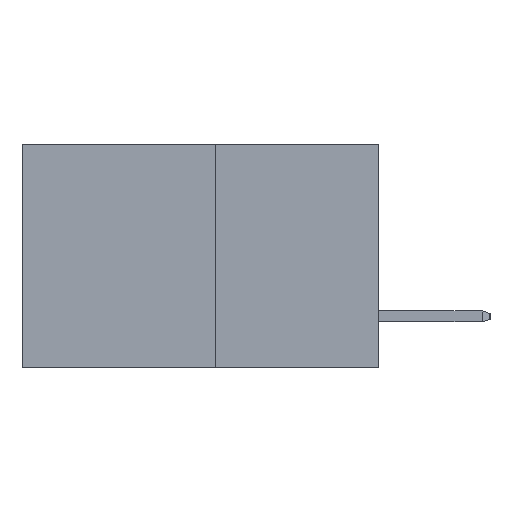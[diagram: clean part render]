
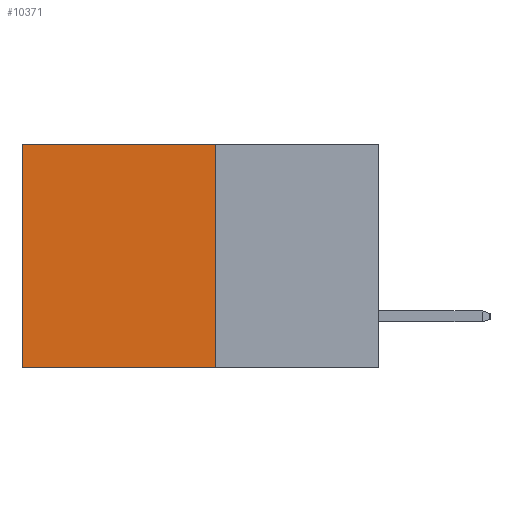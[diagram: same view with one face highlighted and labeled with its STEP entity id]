
A CAD part, left-side view. The second image highlights one B-rep face of the part: STEP entity #10371.
In plain terms, the highlighted planar face has unit normal (-1, 0, 0).
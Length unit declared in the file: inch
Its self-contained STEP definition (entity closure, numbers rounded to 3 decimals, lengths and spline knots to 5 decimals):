
#723 = EDGE_CURVE ( 'NONE', #2415, #3083, #956, .T. ) ;
#948 = VECTOR ( 'NONE', #29250, 39.37008 ) ;
#956 = LINE ( 'NONE', #12950, #25061 ) ;
#1853 = LINE ( 'NONE', #28857, #13525 ) ;
#2415 = VERTEX_POINT ( 'NONE', #9059 ) ;
#3083 = VERTEX_POINT ( 'NONE', #21049 ) ;
#4936 = VECTOR ( 'NONE', #27880, 39.37008 ) ;
#6704 = CARTESIAN_POINT ( 'NONE',  ( 0.277, 0.59, 0. ) ) ;
#7209 = LINE ( 'NONE', #13039, #948 ) ;
#7729 = AXIS2_PLACEMENT_3D ( 'NONE', #22848, #27478, #13544 ) ;
#8076 = DIRECTION ( 'NONE',  ( 0., 1., 0. ) ) ;
#9059 = CARTESIAN_POINT ( 'NONE',  ( 0.277, 0.27, -0.37 ) ) ;
#10371 = ADVANCED_FACE ( 'NONE', ( #15205 ), #25162, .F. ) ;
#12941 = EDGE_CURVE ( 'NONE', #22743, #3083, #7209, .T. ) ;
#12950 = CARTESIAN_POINT ( 'NONE',  ( 0.277, 0.27, -0.37 ) ) ;
#13039 = CARTESIAN_POINT ( 'NONE',  ( 0.277, 0.59, -0.37 ) ) ;
#13525 = VECTOR ( 'NONE', #8076, 39.37008 ) ;
#13544 = DIRECTION ( 'NONE',  ( 0., 0., -1. ) ) ;
#14263 = VERTEX_POINT ( 'NONE', #22163 ) ;
#15205 = FACE_OUTER_BOUND ( 'NONE', #19931, .T. ) ;
#15878 = ORIENTED_EDGE ( 'NONE', *, *, #12941, .T. ) ;
#16720 = EDGE_CURVE ( 'NONE', #14263, #2415, #29609, .T. ) ;
#18840 = ORIENTED_EDGE ( 'NONE', *, *, #723, .F. ) ;
#19029 = ORIENTED_EDGE ( 'NONE', *, *, #29867, .T. ) ;
#19931 = EDGE_LOOP ( 'NONE', ( #15878, #18840, #26506, #19029 ) ) ;
#21049 = CARTESIAN_POINT ( 'NONE',  ( 0.277, 0.59, -0.37 ) ) ;
#22163 = CARTESIAN_POINT ( 'NONE',  ( 0.277, 0.27, 0. ) ) ;
#22552 = DIRECTION ( 'NONE',  ( 0., 1., 0. ) ) ;
#22743 = VERTEX_POINT ( 'NONE', #6704 ) ;
#22848 = CARTESIAN_POINT ( 'NONE',  ( 0.277, 0.27, -0.37 ) ) ;
#25061 = VECTOR ( 'NONE', #22552, 39.37008 ) ;
#25162 = PLANE ( 'NONE',  #7729 ) ;
#25607 = CARTESIAN_POINT ( 'NONE',  ( 0.277, 0.27, -0.37 ) ) ;
#26506 = ORIENTED_EDGE ( 'NONE', *, *, #16720, .F. ) ;
#27478 = DIRECTION ( 'NONE',  ( 1., 0., 0. ) ) ;
#27880 = DIRECTION ( 'NONE',  ( 0., 0., -1. ) ) ;
#28857 = CARTESIAN_POINT ( 'NONE',  ( 0.277, 0.27, 0. ) ) ;
#29250 = DIRECTION ( 'NONE',  ( 0., 0., -1. ) ) ;
#29609 = LINE ( 'NONE', #25607, #4936 ) ;
#29867 = EDGE_CURVE ( 'NONE', #14263, #22743, #1853, .T. ) ;
